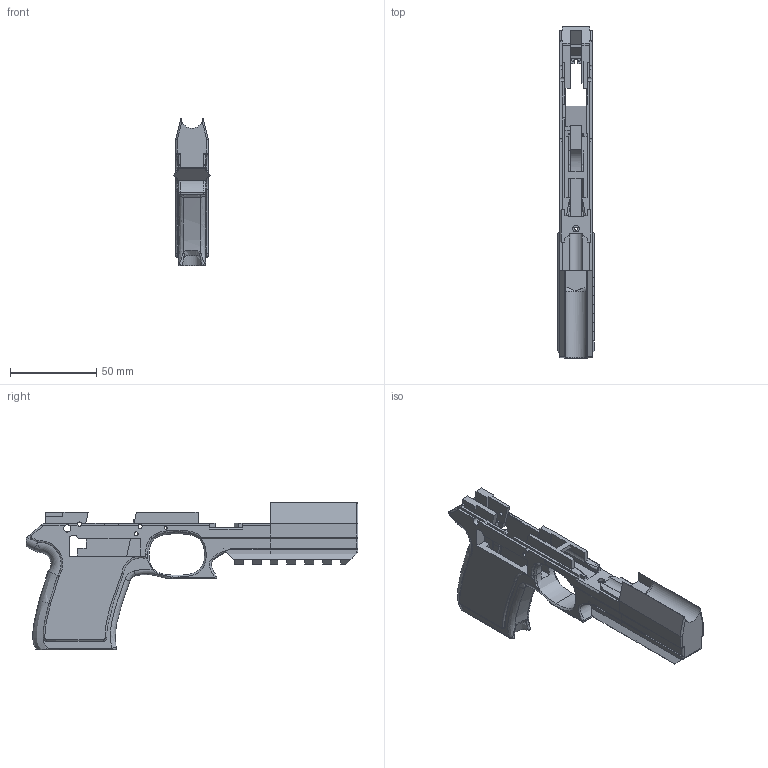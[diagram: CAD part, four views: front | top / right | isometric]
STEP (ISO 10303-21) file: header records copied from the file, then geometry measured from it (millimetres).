
FILE_DESCRIPTION(/* description */ (''),/* implementation_level */ '2;1');
FILE_NAME(/* name */ 'HP22A Target Receiver v7.step',/* time_stamp */ '2020-01-03T17:55:52-05:00',/* author */ (''),/* organization */ (''),/* preprocessor_version */ 'ST-DEVELOPER v18',/* originating_system */ 'Autodesk Translation Framework v8.12.0.6',/* authorisation */ '');
FILE_SCHEMA (('AUTOMOTIVE_DESIGN { 1 0 10303 214 3 1 1 }'));
Length unit declared in the file: millimetre
Products named in the file (1): HP22A Target Receiver
Bounding box: 21.21 x 193 x 85.85 mm (x, y, z)
Volume: 82741.5 mm3; surface area: 36876.3 mm2
Topology: 2 solids, 2 shells, 470 faces, 1317 edges, 835 vertices
Faces by surface type: plane 278, bspline 96, cylinder 77, torus 11, sphere 8
Full cylindrical faces by diameter (mm): 1.5 x2, 1.8 x1, 2.3 x5, 2.45 x2, 3.85 x2, 4.25 x2, 5 x1, 5.7 x1, 5.75 x1
Entity records: 19033 total; most frequent: CARTESIAN_POINT 7465, ORIENTED_EDGE 2634, DIRECTION 2064, EDGE_CURVE 1317, LINE 858, VECTOR 858, VERTEX_POINT 835, AXIS2_PLACEMENT_3D 603
